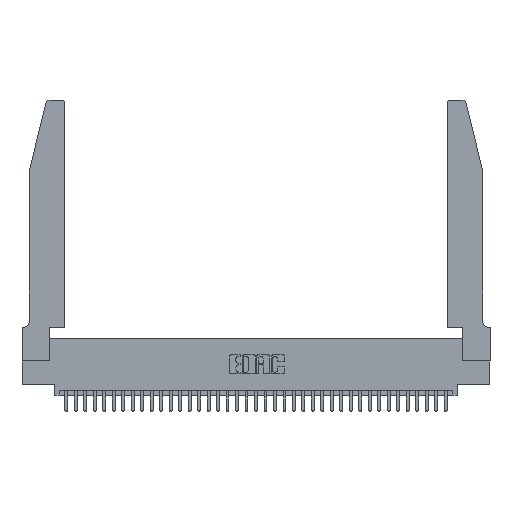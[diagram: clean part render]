
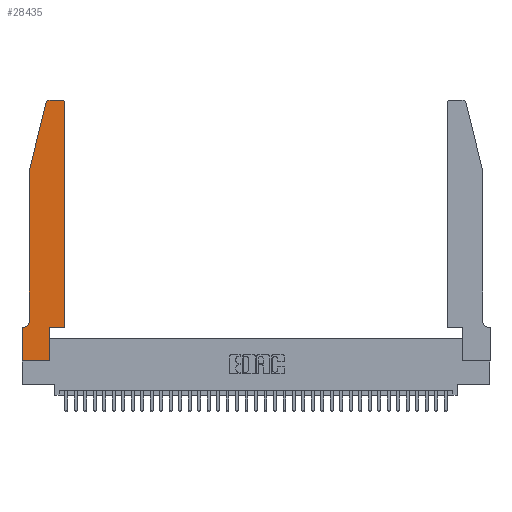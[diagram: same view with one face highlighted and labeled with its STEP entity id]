
A CAD part, top view. The second image highlights one B-rep face of the part: STEP entity #28435.
In plain terms, the highlighted planar face has unit normal (0, 0, 1).
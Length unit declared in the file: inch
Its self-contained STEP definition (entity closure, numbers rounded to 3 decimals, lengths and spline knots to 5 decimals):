
#231 = VECTOR ( 'NONE', #16696, 39.37008 ) ;
#649 = CARTESIAN_POINT ( 'NONE',  ( 0.2605, 2.75, 0.37 ) ) ;
#816 = EDGE_CURVE ( 'NONE', #8899, #24643, #19077, .T. ) ;
#999 = EDGE_CURVE ( 'NONE', #10776, #2677, #13606, .T. ) ;
#1496 = CARTESIAN_POINT ( 'NONE',  ( 0.0755, 2., 0.37 ) ) ;
#2089 = DIRECTION ( 'NONE',  ( -0.239, -0.971, 0. ) ) ;
#2164 = CARTESIAN_POINT ( 'NONE',  ( 0.0755, 2., 0.37 ) ) ;
#2244 = CIRCLE ( 'NONE', #3490, 0.07 ) ;
#2334 = CARTESIAN_POINT ( 'NONE',  ( 0., 0., 0.37 ) ) ;
#2568 = FACE_OUTER_BOUND ( 'NONE', #12711, .T. ) ;
#2677 = VERTEX_POINT ( 'NONE', #21627 ) ;
#2766 = CARTESIAN_POINT ( 'NONE',  ( 0.2865, 0., 0.37 ) ) ;
#2799 = VERTEX_POINT ( 'NONE', #10526 ) ;
#3101 = VERTEX_POINT ( 'NONE', #15067 ) ;
#3465 = EDGE_CURVE ( 'NONE', #3101, #3707, #16859, .T. ) ;
#3490 = AXIS2_PLACEMENT_3D ( 'NONE', #8783, #28985, #11754 ) ;
#3707 = VERTEX_POINT ( 'NONE', #34624 ) ;
#3752 = ORIENTED_EDGE ( 'NONE', *, *, #999, .T. ) ;
#5123 = DIRECTION ( 'NONE',  ( 0., -1., 0. ) ) ;
#6362 = ORIENTED_EDGE ( 'NONE', *, *, #816, .T. ) ;
#6737 = VERTEX_POINT ( 'NONE', #2766 ) ;
#7142 = CARTESIAN_POINT ( 'NONE',  ( 0.0755, 2., 0.37 ) ) ;
#7332 = ORIENTED_EDGE ( 'NONE', *, *, #10756, .T. ) ;
#7340 = CARTESIAN_POINT ( 'NONE',  ( 0.4205, 2.72, 0.37 ) ) ;
#8108 = DIRECTION ( 'NONE',  ( 0., 0., 1. ) ) ;
#8131 = ORIENTED_EDGE ( 'NONE', *, *, #27344, .T. ) ;
#8425 = CARTESIAN_POINT ( 'NONE',  ( 0.284, 2.72, 0.37 ) ) ;
#8783 = CARTESIAN_POINT ( 'NONE',  ( 0.0055, 0.42, 0.37 ) ) ;
#8899 = VERTEX_POINT ( 'NONE', #14451 ) ;
#10139 = LINE ( 'NONE', #21855, #31257 ) ;
#10230 = CARTESIAN_POINT ( 'NONE',  ( 0., 0., 0.37 ) ) ;
#10291 = DIRECTION ( 'NONE',  ( 1., 0., 0. ) ) ;
#10526 = CARTESIAN_POINT ( 'NONE',  ( 0.2865, 0.35, 0.37 ) ) ;
#10756 = EDGE_CURVE ( 'NONE', #24643, #11134, #30618, .T. ) ;
#10776 = VERTEX_POINT ( 'NONE', #16989 ) ;
#10919 = CARTESIAN_POINT ( 'NONE',  ( 0., 0.35, 0.37 ) ) ;
#10987 = CARTESIAN_POINT ( 'NONE',  ( 0., 0., 0.37 ) ) ;
#11134 = VERTEX_POINT ( 'NONE', #33085 ) ;
#11385 = DIRECTION ( 'NONE',  ( 1., 0., 0. ) ) ;
#11754 = DIRECTION ( 'NONE',  ( -1., 0., 0. ) ) ;
#11794 = CARTESIAN_POINT ( 'NONE',  ( 0.4505, 0.35, 0.37 ) ) ;
#12064 = DIRECTION ( 'NONE',  ( 0., 1., 0. ) ) ;
#12519 = AXIS2_PLACEMENT_3D ( 'NONE', #7340, #27593, #10291 ) ;
#12711 = EDGE_LOOP ( 'NONE', ( #26559, #28767, #6362, #7332, #28758, #26502, #24090, #8131, #26690, #13136, #3752, #31202 ) ) ;
#13136 = ORIENTED_EDGE ( 'NONE', *, *, #25916, .T. ) ;
#13606 = LINE ( 'NONE', #11794, #27962 ) ;
#14451 = CARTESIAN_POINT ( 'NONE',  ( 0.25487, 2.72718, 0.37 ) ) ;
#14965 = VECTOR ( 'NONE', #29686, 39.37008 ) ;
#15067 = CARTESIAN_POINT ( 'NONE',  ( 0.0055, 0.35, 0.37 ) ) ;
#16252 = CIRCLE ( 'NONE', #32353, 0.03 ) ;
#16696 = DIRECTION ( 'NONE',  ( -1., 0., 0. ) ) ;
#16859 = LINE ( 'NONE', #33547, #231 ) ;
#16989 = CARTESIAN_POINT ( 'NONE',  ( 0.4505, 0.35, 0.37 ) ) ;
#17354 = CARTESIAN_POINT ( 'NONE',  ( 0.2865, 0.35, 0.37 ) ) ;
#17876 = EDGE_CURVE ( 'NONE', #32165, #8899, #16252, .T. ) ;
#18480 = CARTESIAN_POINT ( 'NONE',  ( 0.4205, 2.75, 0.37 ) ) ;
#19077 = LINE ( 'NONE', #1496, #33254 ) ;
#21627 = CARTESIAN_POINT ( 'NONE',  ( 0.4505, 2.72, 0.37 ) ) ;
#21855 = CARTESIAN_POINT ( 'NONE',  ( 0.4505, 0.35, 0.37 ) ) ;
#22196 = VECTOR ( 'NONE', #34046, 39.37008 ) ;
#22210 = VECTOR ( 'NONE', #5123, 39.37008 ) ;
#22599 = LINE ( 'NONE', #649, #14965 ) ;
#22758 = DIRECTION ( 'NONE',  ( 1., 0., 0. ) ) ;
#24090 = ORIENTED_EDGE ( 'NONE', *, *, #36425, .T. ) ;
#24253 = EDGE_CURVE ( 'NONE', #6737, #2799, #34455, .T. ) ;
#24526 = VECTOR ( 'NONE', #22758, 39.37008 ) ;
#24643 = VERTEX_POINT ( 'NONE', #7142 ) ;
#24662 = VERTEX_POINT ( 'NONE', #10230 ) ;
#25888 = AXIS2_PLACEMENT_3D ( 'NONE', #10919, #8108, #28336 ) ;
#25905 = DIRECTION ( 'NONE',  ( 0., 1., 0. ) ) ;
#25916 = EDGE_CURVE ( 'NONE', #2799, #10776, #10139, .T. ) ;
#26187 = CARTESIAN_POINT ( 'NONE',  ( 0.284, 2.75, 0.37 ) ) ;
#26502 = ORIENTED_EDGE ( 'NONE', *, *, #3465, .T. ) ;
#26559 = ORIENTED_EDGE ( 'NONE', *, *, #37066, .T. ) ;
#26690 = ORIENTED_EDGE ( 'NONE', *, *, #24253, .T. ) ;
#26808 = EDGE_CURVE ( 'NONE', #11134, #3101, #2244, .T. ) ;
#27344 = EDGE_CURVE ( 'NONE', #24662, #6737, #30278, .T. ) ;
#27593 = DIRECTION ( 'NONE',  ( 0., 0., 1. ) ) ;
#27962 = VECTOR ( 'NONE', #12064, 39.37008 ) ;
#28336 = DIRECTION ( 'NONE',  ( 1., 0., 0. ) ) ;
#28435 = ADVANCED_FACE ( 'NONE', ( #2568 ), #36682, .T. ) ;
#28640 = DIRECTION ( 'NONE',  ( 0., 0., 1. ) ) ;
#28758 = ORIENTED_EDGE ( 'NONE', *, *, #26808, .T. ) ;
#28767 = ORIENTED_EDGE ( 'NONE', *, *, #17876, .T. ) ;
#28985 = DIRECTION ( 'NONE',  ( 0., 0., -1. ) ) ;
#29686 = DIRECTION ( 'NONE',  ( -1., 0., 0. ) ) ;
#30278 = LINE ( 'NONE', #2334, #24526 ) ;
#30390 = DIRECTION ( 'NONE',  ( 1., 0., 0. ) ) ;
#30618 = LINE ( 'NONE', #2164, #22210 ) ;
#31202 = ORIENTED_EDGE ( 'NONE', *, *, #33674, .T. ) ;
#31257 = VECTOR ( 'NONE', #30390, 39.37008 ) ;
#32165 = VERTEX_POINT ( 'NONE', #26187 ) ;
#32353 = AXIS2_PLACEMENT_3D ( 'NONE', #8425, #28640, #11385 ) ;
#33085 = CARTESIAN_POINT ( 'NONE',  ( 0.0755, 0.42, 0.37 ) ) ;
#33254 = VECTOR ( 'NONE', #2089, 39.37008 ) ;
#33547 = CARTESIAN_POINT ( 'NONE',  ( 0.0755, 0.35, 0.37 ) ) ;
#33591 = VECTOR ( 'NONE', #25905, 39.37008 ) ;
#33674 = EDGE_CURVE ( 'NONE', #2677, #36028, #33829, .T. ) ;
#33829 = CIRCLE ( 'NONE', #12519, 0.03 ) ;
#34046 = DIRECTION ( 'NONE',  ( 0., -1., 0. ) ) ;
#34455 = LINE ( 'NONE', #17354, #33591 ) ;
#34624 = CARTESIAN_POINT ( 'NONE',  ( 0., 0.35, 0.37 ) ) ;
#36028 = VERTEX_POINT ( 'NONE', #18480 ) ;
#36425 = EDGE_CURVE ( 'NONE', #3707, #24662, #37191, .T. ) ;
#36682 = PLANE ( 'NONE',  #25888 ) ;
#37066 = EDGE_CURVE ( 'NONE', #36028, #32165, #22599, .T. ) ;
#37191 = LINE ( 'NONE', #10987, #22196 ) ;
